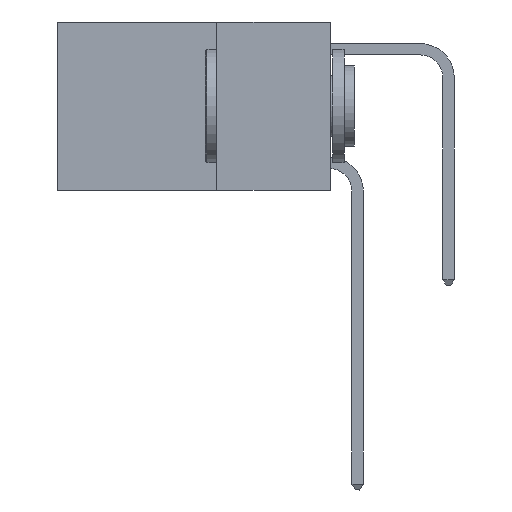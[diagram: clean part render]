
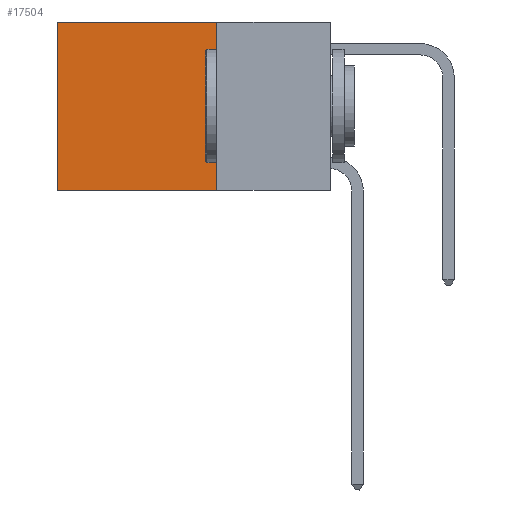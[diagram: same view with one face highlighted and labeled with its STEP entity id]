
A CAD part, left-side view. The second image highlights one B-rep face of the part: STEP entity #17504.
In plain terms, the highlighted planar face has unit normal (-1, 0, 0).
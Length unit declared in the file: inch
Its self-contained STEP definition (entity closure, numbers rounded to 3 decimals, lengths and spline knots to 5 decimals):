
#178 = AXIS2_PLACEMENT_3D ( 'NONE', #25937, #7428, #21622 ) ;
#785 = LINE ( 'NONE', #13262, #19224 ) ;
#1187 = VECTOR ( 'NONE', #12213, 39.37008 ) ;
#1804 = CARTESIAN_POINT ( 'NONE',  ( 0.2625, 0.25, 0. ) ) ;
#3910 = VECTOR ( 'NONE', #4185, 39.37008 ) ;
#3985 = LINE ( 'NONE', #16547, #6504 ) ;
#4185 = DIRECTION ( 'NONE',  ( 0., 1., 0. ) ) ;
#6346 = VERTEX_POINT ( 'NONE', #23801 ) ;
#6504 = VECTOR ( 'NONE', #21360, 39.37008 ) ;
#7428 = DIRECTION ( 'NONE',  ( 1., 0., 0. ) ) ;
#11756 = VERTEX_POINT ( 'NONE', #29587 ) ;
#11769 = ORIENTED_EDGE ( 'NONE', *, *, #23193, .F. ) ;
#12213 = DIRECTION ( 'NONE',  ( 0., 1., 0. ) ) ;
#12364 = ORIENTED_EDGE ( 'NONE', *, *, #18137, .T. ) ;
#12811 = ORIENTED_EDGE ( 'NONE', *, *, #29774, .T. ) ;
#13262 = CARTESIAN_POINT ( 'NONE',  ( 0.2625, 0.25, 0. ) ) ;
#13466 = LINE ( 'NONE', #18836, #1187 ) ;
#14992 = VERTEX_POINT ( 'NONE', #20658 ) ;
#16547 = CARTESIAN_POINT ( 'NONE',  ( 0.2625, 0.6, 0. ) ) ;
#17504 = ADVANCED_FACE ( 'NONE', ( #22434 ), #26038, .F. ) ;
#18137 = EDGE_CURVE ( 'NONE', #29192, #6346, #21667, .T. ) ;
#18836 = CARTESIAN_POINT ( 'NONE',  ( 0.2625, 0.25, -0.37 ) ) ;
#19224 = VECTOR ( 'NONE', #22596, 39.37008 ) ;
#20658 = CARTESIAN_POINT ( 'NONE',  ( 0.2625, 0.25, -0.37 ) ) ;
#21360 = DIRECTION ( 'NONE',  ( 0., 0., -1. ) ) ;
#21622 = DIRECTION ( 'NONE',  ( 0., 0., -1. ) ) ;
#21667 = LINE ( 'NONE', #1804, #3910 ) ;
#22434 = FACE_OUTER_BOUND ( 'NONE', #24070, .T. ) ;
#22596 = DIRECTION ( 'NONE',  ( 0., 0., -1. ) ) ;
#23193 = EDGE_CURVE ( 'NONE', #14992, #11756, #13466, .T. ) ;
#23390 = ORIENTED_EDGE ( 'NONE', *, *, #23676, .F. ) ;
#23676 = EDGE_CURVE ( 'NONE', #29192, #14992, #785, .T. ) ;
#23801 = CARTESIAN_POINT ( 'NONE',  ( 0.2625, 0.6, 0. ) ) ;
#24070 = EDGE_LOOP ( 'NONE', ( #12811, #11769, #23390, #12364 ) ) ;
#25937 = CARTESIAN_POINT ( 'NONE',  ( 0.2625, 0.25, 0. ) ) ;
#26038 = PLANE ( 'NONE',  #178 ) ;
#29010 = CARTESIAN_POINT ( 'NONE',  ( 0.2625, 0.25, 0. ) ) ;
#29192 = VERTEX_POINT ( 'NONE', #29010 ) ;
#29587 = CARTESIAN_POINT ( 'NONE',  ( 0.2625, 0.6, -0.37 ) ) ;
#29774 = EDGE_CURVE ( 'NONE', #6346, #11756, #3985, .T. ) ;
